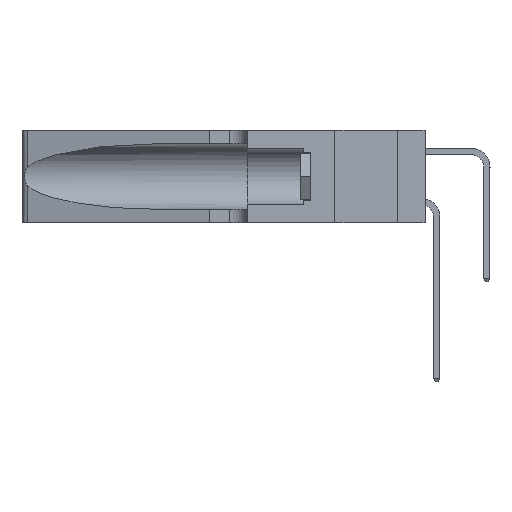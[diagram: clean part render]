
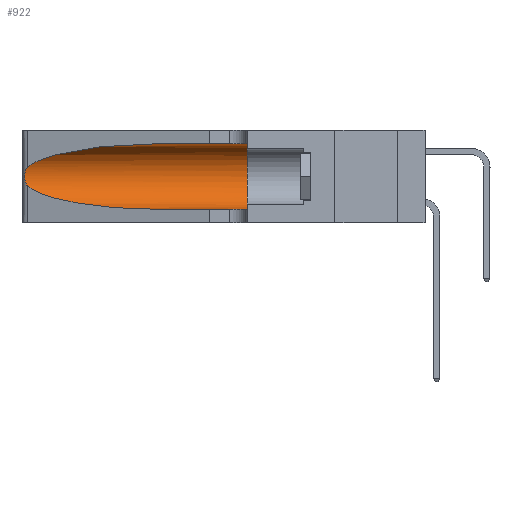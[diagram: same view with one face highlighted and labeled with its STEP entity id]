
A CAD part, left-side view. The second image highlights one B-rep face of the part: STEP entity #922.
In plain terms, the highlighted cylindrical face has radius 3.308 mm (diameter 6.617 mm), a partial arc.
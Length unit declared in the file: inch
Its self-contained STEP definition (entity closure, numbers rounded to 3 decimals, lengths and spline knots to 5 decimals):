
#922 = ADVANCED_FACE ( 'NONE', ( #16480 ), #27836, .F. ) ;
#1040 = CARTESIAN_POINT ( 'NONE',  ( 0.1305, 0.35, 0.185 ) ) ;
#1090 = CARTESIAN_POINT ( 'NONE',  ( 0.18966, 0.96281, 0.05475 ) ) ;
#1571 = CARTESIAN_POINT ( 'NONE',  ( 0.26018, 1.23835, 0.19895 ) ) ;
#2014 = VERTEX_POINT ( 'NONE', #29219 ) ;
#2130 = VERTEX_POINT ( 'NONE', #27843 ) ;
#2457 = ORIENTED_EDGE ( 'NONE', *, *, #20066, .F. ) ;
#3266 = ORIENTED_EDGE ( 'NONE', *, *, #11374, .T. ) ;
#3676 = CARTESIAN_POINT ( 'NONE',  ( 0.25856, 1.23593, 0.16098 ) ) ;
#3892 = CARTESIAN_POINT ( 'NONE',  ( 0.1305, 0.72297, 0.05475 ) ) ;
#4073 = CARTESIAN_POINT ( 'NONE',  ( 0.26017, 1.23833, 0.17102 ) ) ;
#4152 = EDGE_CURVE ( 'NONE', #29602, #2130, #7724, .T. ) ;
#4314 = ORIENTED_EDGE ( 'NONE', *, *, #23695, .T. ) ;
#4635 =( BOUNDED_CURVE ( )  B_SPLINE_CURVE ( 3, ( #19938, #13179, #1090, #24573 ),
 .UNSPECIFIED., .F., .T. ) 
 B_SPLINE_CURVE_WITH_KNOTS ( ( 4, 4 ),
 ( 3.44316, 4.71239 ),
 .UNSPECIFIED. ) 
 CURVE ( )  GEOMETRIC_REPRESENTATION_ITEM ( )  RATIONAL_B_SPLINE_CURVE ( ( 1., 0.87, 0.87, 1. ) ) 
 REPRESENTATION_ITEM ( '' )  );
#5746 = LINE ( 'NONE', #27673, #6918 ) ;
#5990 = B_SPLINE_CURVE_WITH_KNOTS ( 'NONE', 3,
 ( #22412, #20126, #25258, #20330, #25044, #1571, #13159, #29581, #4073, #3676, #6277, #22711, #29797, #8750 ),
 .UNSPECIFIED., .F., .F.,
 ( 4, 2, 2, 2, 2, 2, 4 ),
 ( 0., 0.00027, 0.00053, 0.00107, 0.0016, 0.00187, 0.00214 ),
 .UNSPECIFIED. ) ;
#6111 = AXIS2_PLACEMENT_3D ( 'NONE', #10797, #29685, #11417 ) ;
#6277 = CARTESIAN_POINT ( 'NONE',  ( 0.25789, 1.23486, 0.15765 ) ) ;
#6748 = DIRECTION ( 'NONE',  ( 0., 0., 1. ) ) ;
#6918 = VECTOR ( 'NONE', #13720, 39.37008 ) ;
#7050 = CARTESIAN_POINT ( 'NONE',  ( 0.25487, 1.22718, 0.22369 ) ) ;
#7571 = LINE ( 'NONE', #17107, #15293 ) ;
#7575 = DIRECTION ( 'NONE',  ( 0., -1., 0. ) ) ;
#7654 = AXIS2_PLACEMENT_3D ( 'NONE', #1040, #29551, #6748 ) ;
#7724 =( BOUNDED_CURVE ( )  B_SPLINE_CURVE ( 3, ( #15874, #23847, #25715, #7050 ),
 .UNSPECIFIED., .F., .T. ) 
 B_SPLINE_CURVE_WITH_KNOTS ( ( 4, 4 ),
 ( 1.5708, 2.84003 ),
 .UNSPECIFIED. ) 
 CURVE ( )  GEOMETRIC_REPRESENTATION_ITEM ( )  RATIONAL_B_SPLINE_CURVE ( ( 1., 0.87, 0.87, 1. ) ) 
 REPRESENTATION_ITEM ( '' )  );
#7894 = ORIENTED_EDGE ( 'NONE', *, *, #20393, .F. ) ;
#8750 = CARTESIAN_POINT ( 'NONE',  ( 0.25487, 1.22718, 0.14631 ) ) ;
#10797 = CARTESIAN_POINT ( 'NONE',  ( 0.1305, 1.61858, 0.185 ) ) ;
#11374 = EDGE_CURVE ( 'NONE', #2130, #29439, #5990, .T. ) ;
#11417 = DIRECTION ( 'NONE',  ( 0., 0., -1. ) ) ;
#13159 = CARTESIAN_POINT ( 'NONE',  ( 0.26075, 1.23896, 0.19203 ) ) ;
#13179 = CARTESIAN_POINT ( 'NONE',  ( 0.2373, 1.15595, 0.08982 ) ) ;
#13202 = CARTESIAN_POINT ( 'NONE',  ( 0.1305, 0.35, 0.05475 ) ) ;
#13720 = DIRECTION ( 'NONE',  ( 0., -1., 0. ) ) ;
#14848 = EDGE_CURVE ( 'NONE', #29439, #28414, #4635, .T. ) ;
#15293 = VECTOR ( 'NONE', #7575, 39.37008 ) ;
#15874 = CARTESIAN_POINT ( 'NONE',  ( 0.1305, 0.72297, 0.31525 ) ) ;
#16480 = FACE_OUTER_BOUND ( 'NONE', #21501, .T. ) ;
#17107 = CARTESIAN_POINT ( 'NONE',  ( 0.1305, 1.61858, 0.05475 ) ) ;
#19938 = CARTESIAN_POINT ( 'NONE',  ( 0.25487, 1.22718, 0.14631 ) ) ;
#20066 = EDGE_CURVE ( 'NONE', #29602, #2014, #5746, .T. ) ;
#20126 = CARTESIAN_POINT ( 'NONE',  ( 0.25555, 1.22994, 0.2215 ) ) ;
#20330 = CARTESIAN_POINT ( 'NONE',  ( 0.25787, 1.23484, 0.2124 ) ) ;
#20393 = EDGE_CURVE ( 'NONE', #2014, #26331, #23395, .T. ) ;
#20858 = ORIENTED_EDGE ( 'NONE', *, *, #14848, .T. ) ;
#20922 = ORIENTED_EDGE ( 'NONE', *, *, #4152, .T. ) ;
#21501 = EDGE_LOOP ( 'NONE', ( #20922, #3266, #20858, #4314, #7894, #2457 ) ) ;
#21525 = CARTESIAN_POINT ( 'NONE',  ( 0.1305, 0.72297, 0.31525 ) ) ;
#22412 = CARTESIAN_POINT ( 'NONE',  ( 0.25487, 1.22718, 0.22369 ) ) ;
#22711 = CARTESIAN_POINT ( 'NONE',  ( 0.25639, 1.23186, 0.15144 ) ) ;
#23395 = CIRCLE ( 'NONE', #7654, 0.13025 ) ;
#23695 = EDGE_CURVE ( 'NONE', #28414, #26331, #7571, .T. ) ;
#23847 = CARTESIAN_POINT ( 'NONE',  ( 0.18966, 0.96281, 0.31525 ) ) ;
#24573 = CARTESIAN_POINT ( 'NONE',  ( 0.1305, 0.72297, 0.05475 ) ) ;
#25044 = CARTESIAN_POINT ( 'NONE',  ( 0.25854, 1.2359, 0.20912 ) ) ;
#25258 = CARTESIAN_POINT ( 'NONE',  ( 0.25639, 1.23184, 0.21858 ) ) ;
#25453 = CARTESIAN_POINT ( 'NONE',  ( 0.25487, 1.22718, 0.14631 ) ) ;
#25715 = CARTESIAN_POINT ( 'NONE',  ( 0.2373, 1.15595, 0.28018 ) ) ;
#26331 = VERTEX_POINT ( 'NONE', #13202 ) ;
#27673 = CARTESIAN_POINT ( 'NONE',  ( 0.1305, 1.61858, 0.31525 ) ) ;
#27836 = CYLINDRICAL_SURFACE ( 'NONE', #6111, 0.13025 ) ;
#27843 = CARTESIAN_POINT ( 'NONE',  ( 0.25487, 1.22718, 0.22369 ) ) ;
#28414 = VERTEX_POINT ( 'NONE', #3892 ) ;
#29219 = CARTESIAN_POINT ( 'NONE',  ( 0.1305, 0.35, 0.31525 ) ) ;
#29439 = VERTEX_POINT ( 'NONE', #25453 ) ;
#29551 = DIRECTION ( 'NONE',  ( 0., 1., 0. ) ) ;
#29581 = CARTESIAN_POINT ( 'NONE',  ( 0.26075, 1.23896, 0.178 ) ) ;
#29602 = VERTEX_POINT ( 'NONE', #21525 ) ;
#29685 = DIRECTION ( 'NONE',  ( 0., -1., 0. ) ) ;
#29797 = CARTESIAN_POINT ( 'NONE',  ( 0.25555, 1.22993, 0.14849 ) ) ;
